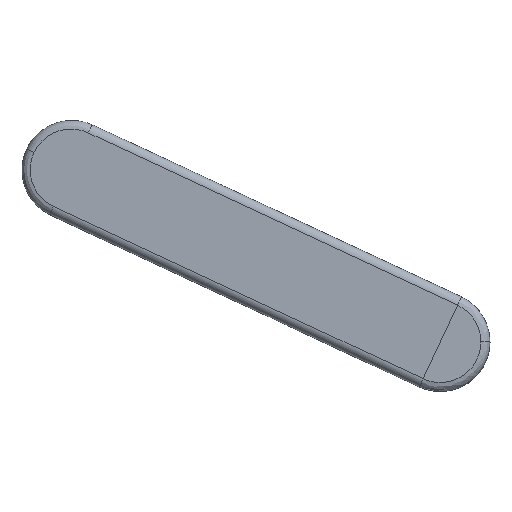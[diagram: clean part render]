
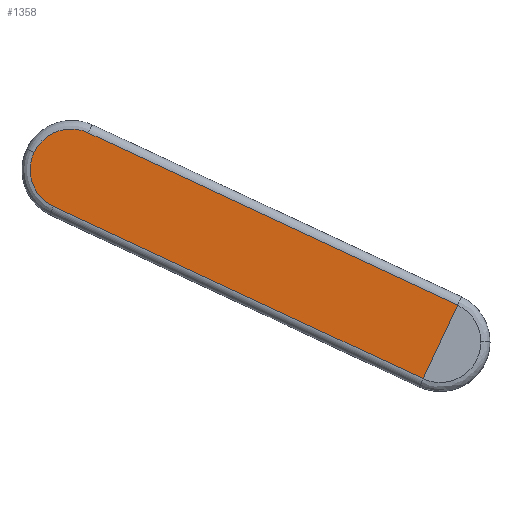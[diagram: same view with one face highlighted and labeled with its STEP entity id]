
A CAD part, top view. The second image highlights one B-rep face of the part: STEP entity #1358.
In plain terms, the highlighted planar face has unit normal (-0.1, 0.047, 0.994).
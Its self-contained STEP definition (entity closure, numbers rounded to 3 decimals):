
#22 = EDGE_LOOP ( 'NONE', ( #76, #1055, #1279, #134, #806 ) ) ;
#52 = VERTEX_POINT ( 'NONE', #667 ) ;
#76 = ORIENTED_EDGE ( 'NONE', *, *, #751, .F. ) ;
#83 = CARTESIAN_POINT ( 'NONE',  ( -4.541, 0.83, 15.004 ) ) ;
#86 = CARTESIAN_POINT ( 'NONE',  ( 18.563, -13.621, 18.009 ) ) ;
#94 = CARTESIAN_POINT ( 'NONE',  ( -0.198, 4.555, 15.266 ) ) ;
#120 = AXIS2_PLACEMENT_3D ( 'NONE', #419, #298, #657 ) ;
#128 = LINE ( 'NONE', #86, #382 ) ;
#134 = ORIENTED_EDGE ( 'NONE', *, *, #862, .T. ) ;
#143 = FACE_OUTER_BOUND ( 'NONE', #22, .T. ) ;
#168 = B_SPLINE_CURVE_WITH_KNOTS ( 'NONE', 3,
 ( #651, #1231, #849, #191, #960, #297, #1050, #417, #1143, #545, #1239, #655, #1333, #763, #83, #854, #195, #965 ),
 .UNSPECIFIED., .F., .F.,
 ( 4, 2, 2, 2, 2, 2, 2, 2, 4 ),
 ( 0., 0.125, 0.25, 0.375, 0.5, 0.625, 0.75, 0.875, 1. ),
 .UNSPECIFIED. ) ;
#185 = VERTEX_POINT ( 'NONE', #676 ) ;
#191 = CARTESIAN_POINT ( 'NONE',  ( -2.998, -3.408, 15.358 ) ) ;
#195 = CARTESIAN_POINT ( 'NONE',  ( -4.303, 1.682, 14.988 ) ) ;
#201 = CARTESIAN_POINT ( 'NONE',  ( 22.366, -5.464, 18.009 ) ) ;
#207 = CARTESIAN_POINT ( 'NONE',  ( 0.683, 4.488, 15.358 ) ) ;
#261 = CARTESIAN_POINT ( 'NONE',  ( 42.686, -14.939, 20.5 ) ) ;
#281 = LINE ( 'NONE', #261, #564 ) ;
#297 = CARTESIAN_POINT ( 'NONE',  ( -3.617, -2.776, 15.266 ) ) ;
#298 = DIRECTION ( 'NONE',  ( 0.1, -0.047, -0.994 ) ) ;
#309 = CARTESIAN_POINT ( 'NONE',  ( -3.555, 2.945, 15.004 ) ) ;
#314 = CARTESIAN_POINT ( 'NONE',  ( 1.535, 4.25, 15.455 ) ) ;
#351 = VECTOR ( 'NONE', #439, 1000. ) ;
#355 = VERTEX_POINT ( 'NONE', #646 ) ;
#366 = DIRECTION ( 'NONE',  ( -0.423, -0.906, 0. ) ) ;
#382 = VECTOR ( 'NONE', #1339, 1000. ) ;
#417 = CARTESIAN_POINT ( 'NONE',  ( -4.1, -2.036, 15.183 ) ) ;
#419 = CARTESIAN_POINT ( 'NONE',  ( 42.931, -23.262, 20.915 ) ) ;
#430 = CARTESIAN_POINT ( 'NONE',  ( -2.923, 3.563, 15.038 ) ) ;
#439 = DIRECTION ( 'NONE',  ( -0.901, 0.42, -0.11 ) ) ;
#514 = CARTESIAN_POINT ( 'NONE',  ( 42.686, -14.939, 20.5 ) ) ;
#545 = CARTESIAN_POINT ( 'NONE',  ( -4.429, -1.216, 15.111 ) ) ;
#559 = CARTESIAN_POINT ( 'NONE',  ( -2.183, 4.047, 15.09 ) ) ;
#564 = VECTOR ( 'NONE', #366, 1000. ) ;
#598 = B_SPLINE_CURVE_WITH_KNOTS ( 'NONE', 3,
 ( #1277, #1058, #969, #309, #1060, #430, #1156, #559, #1252, #665, #1345, #772, #94, #867, #207, #974, #314, #1066 ),
 .UNSPECIFIED., .F., .F.,
 ( 4, 2, 2, 2, 2, 2, 2, 2, 4 ),
 ( 0., 0.125, 0.25, 0.375, 0.5, 0.625, 0.75, 0.875, 1. ),
 .UNSPECIFIED. ) ;
#646 = CARTESIAN_POINT ( 'NONE',  ( 38.882, -23.096, 20.5 ) ) ;
#651 = CARTESIAN_POINT ( 'NONE',  ( -2.002, -4.032, 15.488 ) ) ;
#655 = CARTESIAN_POINT ( 'NONE',  ( -4.593, -0.347, 15.054 ) ) ;
#657 = DIRECTION ( 'NONE',  ( -0.995, 0., -0.1 ) ) ;
#665 = CARTESIAN_POINT ( 'NONE',  ( -1.362, 4.376, 15.157 ) ) ;
#667 = CARTESIAN_POINT ( 'NONE',  ( 1.802, 4.125, 15.488 ) ) ;
#676 = CARTESIAN_POINT ( 'NONE',  ( -4.178, 1.948, 14.988 ) ) ;
#751 = EDGE_CURVE ( 'NONE', #753, #185, #168, .T. ) ;
#753 = VERTEX_POINT ( 'NONE', #953 ) ;
#763 = CARTESIAN_POINT ( 'NONE',  ( -4.583, 0.537, 15.013 ) ) ;
#772 = CARTESIAN_POINT ( 'NONE',  ( -0.494, 4.539, 15.237 ) ) ;
#792 = EDGE_CURVE ( 'NONE', #753, #355, #128, .T. ) ;
#806 = ORIENTED_EDGE ( 'NONE', *, *, #856, .F. ) ;
#849 = CARTESIAN_POINT ( 'NONE',  ( -2.523, -3.756, 15.422 ) ) ;
#854 = CARTESIAN_POINT ( 'NONE',  ( -4.401, 1.402, 14.991 ) ) ;
#856 = EDGE_CURVE ( 'NONE', #185, #52, #598, .T. ) ;
#862 = EDGE_CURVE ( 'NONE', #1042, #52, #1184, .T. ) ;
#867 = CARTESIAN_POINT ( 'NONE',  ( 0.39, 4.53, 15.327 ) ) ;
#951 = EDGE_CURVE ( 'NONE', #1042, #355, #281, .T. ) ;
#953 = CARTESIAN_POINT ( 'NONE',  ( -2.002, -4.032, 15.488 ) ) ;
#960 = CARTESIAN_POINT ( 'NONE',  ( -3.219, -3.211, 15.327 ) ) ;
#965 = CARTESIAN_POINT ( 'NONE',  ( -4.178, 1.948, 14.988 ) ) ;
#969 = CARTESIAN_POINT ( 'NONE',  ( -3.903, 2.47, 14.991 ) ) ;
#974 = CARTESIAN_POINT ( 'NONE',  ( 1.256, 4.348, 15.422 ) ) ;
#1042 = VERTEX_POINT ( 'NONE', #514 ) ;
#1050 = CARTESIAN_POINT ( 'NONE',  ( -3.794, -2.54, 15.237 ) ) ;
#1055 = ORIENTED_EDGE ( 'NONE', *, *, #792, .T. ) ;
#1058 = CARTESIAN_POINT ( 'NONE',  ( -4.054, 2.215, 14.988 ) ) ;
#1060 = CARTESIAN_POINT ( 'NONE',  ( -3.357, 3.165, 15.013 ) ) ;
#1066 = CARTESIAN_POINT ( 'NONE',  ( 1.802, 4.125, 15.488 ) ) ;
#1143 = CARTESIAN_POINT ( 'NONE',  ( -4.228, -1.769, 15.157 ) ) ;
#1156 = CARTESIAN_POINT ( 'NONE',  ( -2.686, 3.741, 15.054 ) ) ;
#1184 = LINE ( 'NONE', #201, #351 ) ;
#1231 = CARTESIAN_POINT ( 'NONE',  ( -2.269, -3.907, 15.455 ) ) ;
#1239 = CARTESIAN_POINT ( 'NONE',  ( -4.503, -0.929, 15.09 ) ) ;
#1240 = PLANE ( 'NONE',  #120 ) ;
#1252 = CARTESIAN_POINT ( 'NONE',  ( -1.916, 4.175, 15.111 ) ) ;
#1277 = CARTESIAN_POINT ( 'NONE',  ( -4.178, 1.948, 14.988 ) ) ;
#1279 = ORIENTED_EDGE ( 'NONE', *, *, #951, .F. ) ;
#1333 = CARTESIAN_POINT ( 'NONE',  ( -4.609, -0.051, 15.038 ) ) ;
#1339 = DIRECTION ( 'NONE',  ( 0.901, -0.42, 0.11 ) ) ;
#1345 = CARTESIAN_POINT ( 'NONE',  ( -1.076, 4.449, 15.183 ) ) ;
#1358 = ADVANCED_FACE ( 'NONE', ( #143 ), #1240, .F. ) ;
